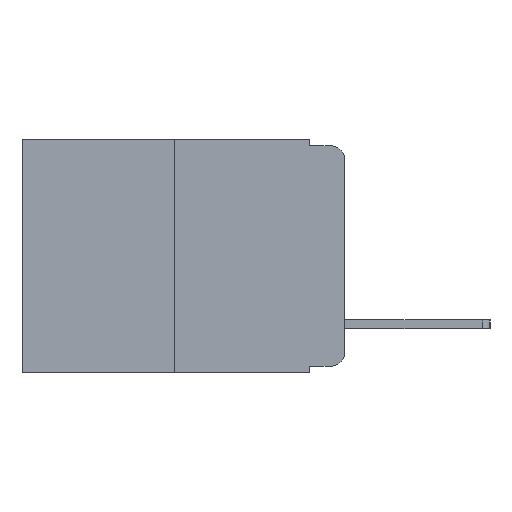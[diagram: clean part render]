
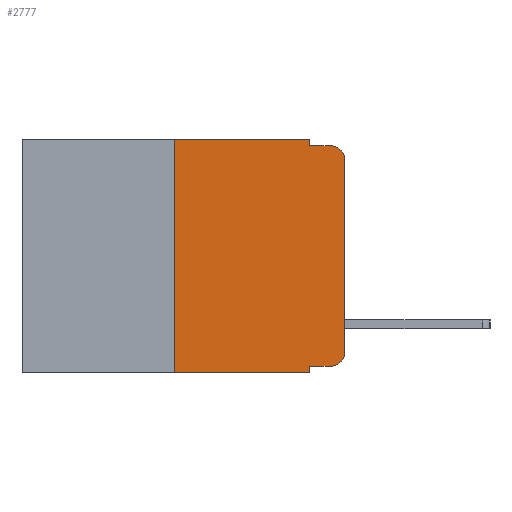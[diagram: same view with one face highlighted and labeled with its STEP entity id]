
A CAD part, left-side view. The second image highlights one B-rep face of the part: STEP entity #2777.
In plain terms, the highlighted planar face has unit normal (-1, 0, 0).
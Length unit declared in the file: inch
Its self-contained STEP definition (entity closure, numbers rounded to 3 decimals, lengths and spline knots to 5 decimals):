
#35 = CARTESIAN_POINT ( 'NONE',  ( 0., 0.051, -0.01 ) ) ;
#449 = CIRCLE ( 'NONE', #1448, 0.02 ) ;
#462 = EDGE_CURVE ( 'NONE', #3052, #4576, #13675, .T. ) ;
#587 = EDGE_CURVE ( 'NONE', #12670, #3052, #7827, .T. ) ;
#628 = VECTOR ( 'NONE', #3211, 39.37008 ) ;
#690 = DIRECTION ( 'NONE',  ( 0., 0., -1. ) ) ;
#1447 = DIRECTION ( 'NONE',  ( 0., 0., -1. ) ) ;
#1448 = AXIS2_PLACEMENT_3D ( 'NONE', #4307, #12420, #12376 ) ;
#1633 = EDGE_CURVE ( 'NONE', #4576, #6524, #8299, .T. ) ;
#1722 = AXIS2_PLACEMENT_3D ( 'NONE', #15662, #9068, #1447 ) ;
#1926 = VERTEX_POINT ( 'NONE', #12405 ) ;
#2572 = EDGE_CURVE ( 'NONE', #6524, #5377, #5145, .T. ) ;
#2581 = CARTESIAN_POINT ( 'NONE',  ( 0., 0.051, 0. ) ) ;
#2777 = ADVANCED_FACE ( 'NONE', ( #8647 ), #7024, .F. ) ;
#3052 = VERTEX_POINT ( 'NONE', #5826 ) ;
#3211 = DIRECTION ( 'NONE',  ( 0., -1., 0. ) ) ;
#3432 = EDGE_CURVE ( 'NONE', #4826, #5377, #449, .T. ) ;
#4162 = CARTESIAN_POINT ( 'NONE',  ( 0., 0.051, -0.333 ) ) ;
#4271 = EDGE_CURVE ( 'NONE', #4723, #4826, #13635, .T. ) ;
#4272 = CARTESIAN_POINT ( 'NONE',  ( 0., 0., -0.313 ) ) ;
#4289 = DIRECTION ( 'NONE',  ( 0., -1., 0. ) ) ;
#4307 = CARTESIAN_POINT ( 'NONE',  ( 0., 0.02, -0.03 ) ) ;
#4486 = LINE ( 'NONE', #13815, #13512 ) ;
#4576 = VERTEX_POINT ( 'NONE', #6458 ) ;
#4723 = VERTEX_POINT ( 'NONE', #4272 ) ;
#4826 = VERTEX_POINT ( 'NONE', #11660 ) ;
#4974 = VECTOR ( 'NONE', #9927, 39.37008 ) ;
#4997 = VECTOR ( 'NONE', #690, 39.37008 ) ;
#5145 = LINE ( 'NONE', #13908, #14074 ) ;
#5361 = DIRECTION ( 'NONE',  ( 0., -1., 0. ) ) ;
#5377 = VERTEX_POINT ( 'NONE', #14846 ) ;
#5444 = CARTESIAN_POINT ( 'NONE',  ( 0., 0.02, -0.333 ) ) ;
#5644 = EDGE_CURVE ( 'NONE', #12670, #13726, #14234, .T. ) ;
#5678 = DIRECTION ( 'NONE',  ( 0., 0., -1. ) ) ;
#5826 = CARTESIAN_POINT ( 'NONE',  ( 0., 0.25, 0. ) ) ;
#5861 = CIRCLE ( 'NONE', #1722, 0.02 ) ;
#6458 = CARTESIAN_POINT ( 'NONE',  ( 0., 0.051, 0. ) ) ;
#6524 = VERTEX_POINT ( 'NONE', #35 ) ;
#6987 = CARTESIAN_POINT ( 'NONE',  ( 0., 0.25, -0.343 ) ) ;
#7024 = PLANE ( 'NONE',  #8924 ) ;
#7576 = VECTOR ( 'NONE', #10690, 39.37008 ) ;
#7665 = VECTOR ( 'NONE', #5361, 39.37008 ) ;
#7703 = VERTEX_POINT ( 'NONE', #5444 ) ;
#7827 = LINE ( 'NONE', #9805, #10575 ) ;
#8299 = LINE ( 'NONE', #2581, #4997 ) ;
#8359 = CARTESIAN_POINT ( 'NONE',  ( 0., 0.473, 0. ) ) ;
#8501 = CARTESIAN_POINT ( 'NONE',  ( 0., 0.051, -0.343 ) ) ;
#8647 = FACE_OUTER_BOUND ( 'NONE', #11517, .T. ) ;
#8741 = CARTESIAN_POINT ( 'NONE',  ( 0., 0.473, -0.343 ) ) ;
#8924 = AXIS2_PLACEMENT_3D ( 'NONE', #10999, #11187, #11199 ) ;
#9046 = ORIENTED_EDGE ( 'NONE', *, *, #13999, .T. ) ;
#9068 = DIRECTION ( 'NONE',  ( -1., 0., 0. ) ) ;
#9805 = CARTESIAN_POINT ( 'NONE',  ( 0., 0.25, 0. ) ) ;
#9927 = DIRECTION ( 'NONE',  ( 0., -1., 0. ) ) ;
#9960 = ORIENTED_EDGE ( 'NONE', *, *, #14704, .T. ) ;
#10575 = VECTOR ( 'NONE', #11268, 39.37008 ) ;
#10690 = DIRECTION ( 'NONE',  ( 0., 0., 1. ) ) ;
#10931 = ORIENTED_EDGE ( 'NONE', *, *, #3432, .T. ) ;
#10999 = CARTESIAN_POINT ( 'NONE',  ( 0., 0.473, 0. ) ) ;
#11066 = ORIENTED_EDGE ( 'NONE', *, *, #4271, .T. ) ;
#11126 = ORIENTED_EDGE ( 'NONE', *, *, #1633, .F. ) ;
#11140 = ORIENTED_EDGE ( 'NONE', *, *, #2572, .F. ) ;
#11187 = DIRECTION ( 'NONE',  ( 1., 0., 0. ) ) ;
#11199 = DIRECTION ( 'NONE',  ( 0., 0., -1. ) ) ;
#11268 = DIRECTION ( 'NONE',  ( 0., 0., 1. ) ) ;
#11423 = ORIENTED_EDGE ( 'NONE', *, *, #462, .F. ) ;
#11517 = EDGE_LOOP ( 'NONE', ( #11066, #10931, #11140, #11126, #11423, #11653, #11639, #11598, #9960, #9046 ) ) ;
#11598 = ORIENTED_EDGE ( 'NONE', *, *, #15428, .F. ) ;
#11639 = ORIENTED_EDGE ( 'NONE', *, *, #5644, .T. ) ;
#11653 = ORIENTED_EDGE ( 'NONE', *, *, #587, .F. ) ;
#11660 = CARTESIAN_POINT ( 'NONE',  ( 0., 0., -0.03 ) ) ;
#12376 = DIRECTION ( 'NONE',  ( 0., 0., -1. ) ) ;
#12405 = CARTESIAN_POINT ( 'NONE',  ( 0., 0.051, -0.333 ) ) ;
#12420 = DIRECTION ( 'NONE',  ( -1., 0., 0. ) ) ;
#12670 = VERTEX_POINT ( 'NONE', #6987 ) ;
#12862 = CARTESIAN_POINT ( 'NONE',  ( 0., 0., 0. ) ) ;
#13512 = VECTOR ( 'NONE', #5678, 39.37008 ) ;
#13635 = LINE ( 'NONE', #12862, #7576 ) ;
#13675 = LINE ( 'NONE', #8359, #628 ) ;
#13704 = LINE ( 'NONE', #4162, #7665 ) ;
#13726 = VERTEX_POINT ( 'NONE', #8501 ) ;
#13815 = CARTESIAN_POINT ( 'NONE',  ( 0., 0.051, 0. ) ) ;
#13908 = CARTESIAN_POINT ( 'NONE',  ( 0., 0.051, -0.01 ) ) ;
#13999 = EDGE_CURVE ( 'NONE', #7703, #4723, #5861, .T. ) ;
#14074 = VECTOR ( 'NONE', #4289, 39.37008 ) ;
#14234 = LINE ( 'NONE', #8741, #4974 ) ;
#14704 = EDGE_CURVE ( 'NONE', #1926, #7703, #13704, .T. ) ;
#14846 = CARTESIAN_POINT ( 'NONE',  ( 0., 0.02, -0.01 ) ) ;
#15428 = EDGE_CURVE ( 'NONE', #1926, #13726, #4486, .T. ) ;
#15662 = CARTESIAN_POINT ( 'NONE',  ( 0., 0.02, -0.313 ) ) ;
